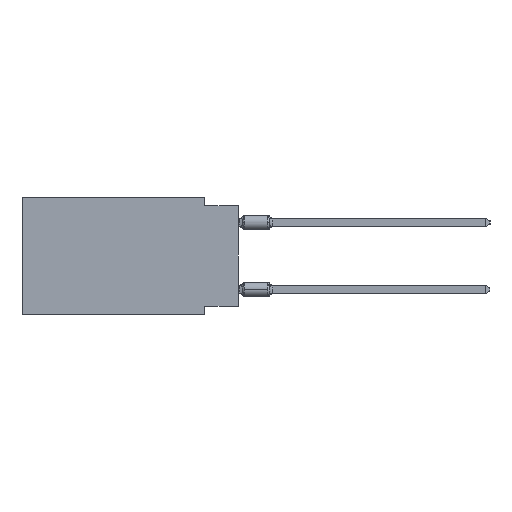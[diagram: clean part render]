
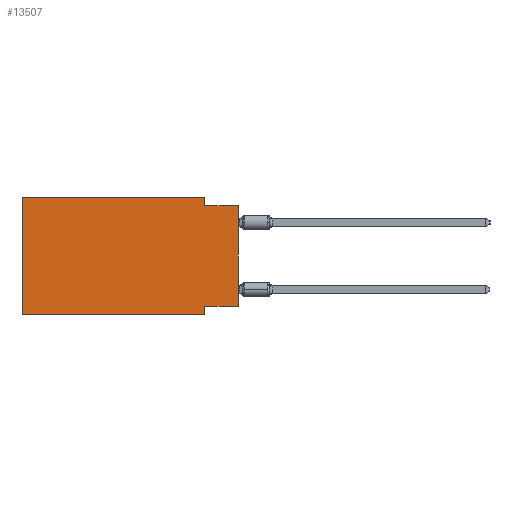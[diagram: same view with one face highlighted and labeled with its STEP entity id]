
A CAD part, left-side view. The second image highlights one B-rep face of the part: STEP entity #13507.
In plain terms, the highlighted planar face has unit normal (-1, 0, 0).
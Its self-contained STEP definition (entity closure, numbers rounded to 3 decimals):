
#184 = EDGE_CURVE ( 'NONE', #21867, #5757, #1404, .T. ) ;
#563 = CARTESIAN_POINT ( 'NONE',  ( 0., 0., -0.635 ) ) ;
#1033 = VECTOR ( 'NONE', #14093, 1000. ) ;
#1286 = VECTOR ( 'NONE', #25837, 1000. ) ;
#1404 = LINE ( 'NONE', #21016, #27626 ) ;
#2907 = VECTOR ( 'NONE', #22747, 1000. ) ;
#2923 = PLANE ( 'NONE',  #21798 ) ;
#3938 = ORIENTED_EDGE ( 'NONE', *, *, #8616, .T. ) ;
#4274 = ORIENTED_EDGE ( 'NONE', *, *, #6715, .F. ) ;
#4604 = ORIENTED_EDGE ( 'NONE', *, *, #6692, .F. ) ;
#4706 = EDGE_LOOP ( 'NONE', ( #3938, #26760, #6593, #17646, #12602, #23172, #4274, #4604 ) ) ;
#5034 = LINE ( 'NONE', #13661, #1033 ) ;
#5110 = CARTESIAN_POINT ( 'NONE',  ( 0., 16.383, 0. ) ) ;
#5351 = CARTESIAN_POINT ( 'NONE',  ( 0., 2.54, -8.255 ) ) ;
#5381 = DIRECTION ( 'NONE',  ( 0., 0., -1. ) ) ;
#5608 = CARTESIAN_POINT ( 'NONE',  ( 0., 16.383, 0. ) ) ;
#5757 = VERTEX_POINT ( 'NONE', #17550 ) ;
#6516 = VERTEX_POINT ( 'NONE', #8539 ) ;
#6593 = ORIENTED_EDGE ( 'NONE', *, *, #184, .F. ) ;
#6692 = EDGE_CURVE ( 'NONE', #23818, #21049, #11891, .T. ) ;
#6715 = EDGE_CURVE ( 'NONE', #21049, #28628, #5034, .T. ) ;
#8539 = CARTESIAN_POINT ( 'NONE',  ( 0., 0., -0.635 ) ) ;
#8616 = EDGE_CURVE ( 'NONE', #23818, #6516, #17632, .T. ) ;
#8802 = VERTEX_POINT ( 'NONE', #12004 ) ;
#9638 = EDGE_CURVE ( 'NONE', #8802, #21867, #12797, .T. ) ;
#9938 = CARTESIAN_POINT ( 'NONE',  ( 0., 2.54, -8.89 ) ) ;
#10074 = CARTESIAN_POINT ( 'NONE',  ( 0., 0., -8.255 ) ) ;
#10413 = LINE ( 'NONE', #5608, #1286 ) ;
#11891 = LINE ( 'NONE', #14226, #2907 ) ;
#12004 = CARTESIAN_POINT ( 'NONE',  ( 0., 16.383, 0. ) ) ;
#12602 = ORIENTED_EDGE ( 'NONE', *, *, #14357, .F. ) ;
#12797 = LINE ( 'NONE', #28216, #15177 ) ;
#13219 = CARTESIAN_POINT ( 'NONE',  ( 0., 0., 0. ) ) ;
#13507 = ADVANCED_FACE ( 'NONE', ( #23408 ), #2923, .F. ) ;
#13661 = CARTESIAN_POINT ( 'NONE',  ( 0., 2.54, -8.89 ) ) ;
#13898 = EDGE_CURVE ( 'NONE', #5757, #6516, #25294, .T. ) ;
#14093 = DIRECTION ( 'NONE',  ( 0., 0., -1. ) ) ;
#14226 = CARTESIAN_POINT ( 'NONE',  ( 0., 0., -8.255 ) ) ;
#14357 = EDGE_CURVE ( 'NONE', #19599, #8802, #10413, .T. ) ;
#14825 = EDGE_CURVE ( 'NONE', #19599, #28628, #26201, .T. ) ;
#15177 = VECTOR ( 'NONE', #26016, 1000. ) ;
#15481 = DIRECTION ( 'NONE',  ( 0., -1., 0. ) ) ;
#16112 = DIRECTION ( 'NONE',  ( 0., 0., 1. ) ) ;
#16721 = VECTOR ( 'NONE', #15481, 1000. ) ;
#17029 = DIRECTION ( 'NONE',  ( 0., 0., -1. ) ) ;
#17550 = CARTESIAN_POINT ( 'NONE',  ( 0., 2.54, -0.635 ) ) ;
#17632 = LINE ( 'NONE', #13219, #28258 ) ;
#17646 = ORIENTED_EDGE ( 'NONE', *, *, #9638, .F. ) ;
#18688 = DIRECTION ( 'NONE',  ( 0., -1., 0. ) ) ;
#19019 = VECTOR ( 'NONE', #18688, 1000. ) ;
#19599 = VERTEX_POINT ( 'NONE', #26907 ) ;
#21016 = CARTESIAN_POINT ( 'NONE',  ( 0., 2.54, 0. ) ) ;
#21049 = VERTEX_POINT ( 'NONE', #5351 ) ;
#21541 = CARTESIAN_POINT ( 'NONE',  ( 0., 2.54, 0. ) ) ;
#21798 = AXIS2_PLACEMENT_3D ( 'NONE', #5110, #27806, #5381 ) ;
#21867 = VERTEX_POINT ( 'NONE', #21541 ) ;
#22747 = DIRECTION ( 'NONE',  ( 0., 1., 0. ) ) ;
#23172 = ORIENTED_EDGE ( 'NONE', *, *, #14825, .T. ) ;
#23408 = FACE_OUTER_BOUND ( 'NONE', #4706, .T. ) ;
#23818 = VERTEX_POINT ( 'NONE', #10074 ) ;
#25294 = LINE ( 'NONE', #563, #19019 ) ;
#25837 = DIRECTION ( 'NONE',  ( 0., 0., 1. ) ) ;
#26016 = DIRECTION ( 'NONE',  ( 0., -1., 0. ) ) ;
#26201 = LINE ( 'NONE', #26482, #16721 ) ;
#26482 = CARTESIAN_POINT ( 'NONE',  ( 0., 16.383, -8.89 ) ) ;
#26760 = ORIENTED_EDGE ( 'NONE', *, *, #13898, .F. ) ;
#26907 = CARTESIAN_POINT ( 'NONE',  ( 0., 16.383, -8.89 ) ) ;
#27626 = VECTOR ( 'NONE', #17029, 1000. ) ;
#27806 = DIRECTION ( 'NONE',  ( 1., 0., 0. ) ) ;
#28216 = CARTESIAN_POINT ( 'NONE',  ( 0., 16.383, 0. ) ) ;
#28258 = VECTOR ( 'NONE', #16112, 1000. ) ;
#28628 = VERTEX_POINT ( 'NONE', #9938 ) ;
